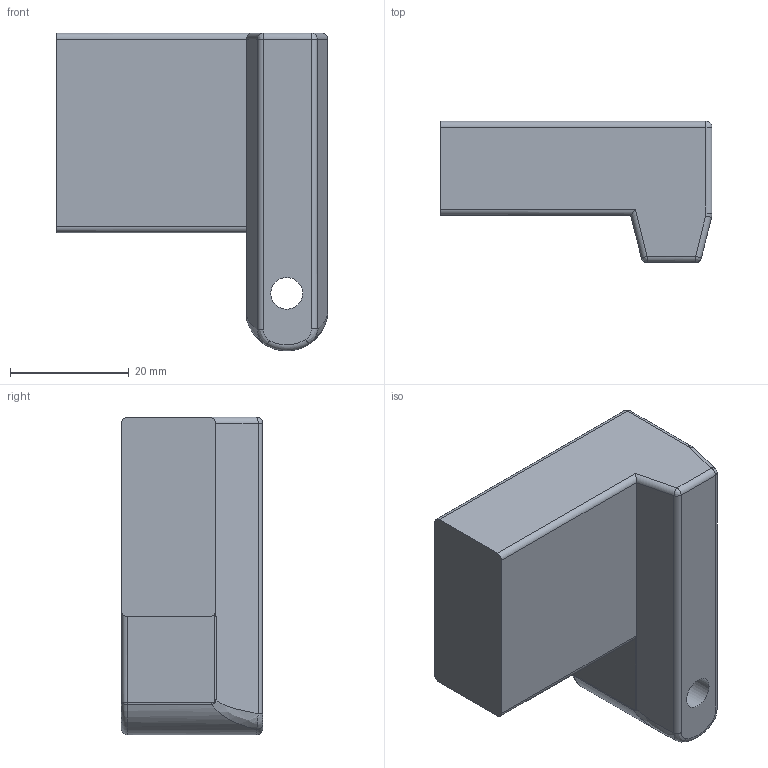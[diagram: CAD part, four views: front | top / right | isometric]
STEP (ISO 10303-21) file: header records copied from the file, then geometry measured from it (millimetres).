
FILE_DESCRIPTION (( 'STEP AP203' ), '1' );
FILE_NAME ('MOD9_stock_lock.STEP', '2020-06-10T05:00:44', ( '' ), ( '' ), 'SwSTEP 2.0', 'SolidWorks 2016', '' );
FILE_SCHEMA (( 'CONFIG_CONTROL_DESIGN' ));
Length unit declared in the file: millimetre
Products named in the file (1): MOD9_stock_lock
Bounding box: 45.75 x 23.76 x 53.45 mm (x, y, z)
Volume: 32558.6 mm3; surface area: 7653.3 mm2
Topology: 1 solids, 1 shells, 43 faces, 103 edges, 59 vertices
Faces by surface type: cylinder 17, plane 13, bspline 7, torus 3, sphere 2, cone 1
Full cylindrical faces by diameter (mm): 5.346 x1
Entity records: 1468 total; most frequent: CARTESIAN_POINT 480, ORIENTED_EDGE 196, DIRECTION 173, EDGE_CURVE 98, AXIS2_PLACEMENT_3D 65, VERTEX_POINT 59, EDGE_LOOP 47, FACE_OUTER_BOUND 44
